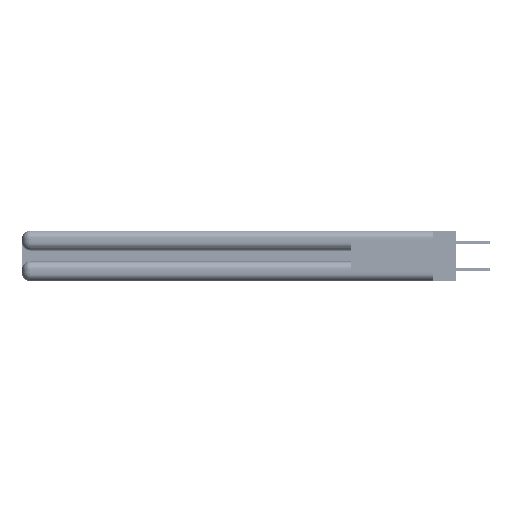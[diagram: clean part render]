
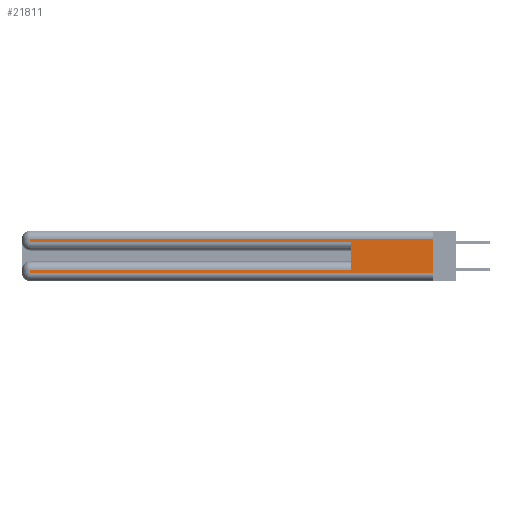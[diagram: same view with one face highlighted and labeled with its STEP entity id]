
A CAD part, left-side view. The second image highlights one B-rep face of the part: STEP entity #21811.
In plain terms, the highlighted planar face has unit normal (-1, 0, 0).
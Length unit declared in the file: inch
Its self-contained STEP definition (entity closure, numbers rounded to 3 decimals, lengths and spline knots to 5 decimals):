
#306 = VERTEX_POINT ( 'NONE', #36244 ) ;
#839 = CARTESIAN_POINT ( 'NONE',  ( 0., 2.94, 0.37 ) ) ;
#999 = VECTOR ( 'NONE', #22378, 39.37008 ) ;
#1964 = EDGE_CURVE ( 'NONE', #41503, #306, #30579, .T. ) ;
#2880 = CARTESIAN_POINT ( 'NONE',  ( 0., 2.94, 0.285 ) ) ;
#4609 = VECTOR ( 'NONE', #44066, 39.37008 ) ;
#4792 = VECTOR ( 'NONE', #18632, 39.37008 ) ;
#5187 = VERTEX_POINT ( 'NONE', #34090 ) ;
#5436 = CARTESIAN_POINT ( 'NONE',  ( 0., 2.94, 0.06 ) ) ;
#5549 = DIRECTION ( 'NONE',  ( 1., 0., 0. ) ) ;
#5707 = PLANE ( 'NONE',  #13235 ) ;
#6032 = EDGE_CURVE ( 'NONE', #41503, #29476, #15359, .T. ) ;
#6185 = FACE_OUTER_BOUND ( 'NONE', #9806, .T. ) ;
#6890 = LINE ( 'NONE', #13464, #4609 ) ;
#7035 = LINE ( 'NONE', #839, #19887 ) ;
#7807 = LINE ( 'NONE', #8711, #35092 ) ;
#8030 = DIRECTION ( 'NONE',  ( 0., 0., -1. ) ) ;
#8711 = CARTESIAN_POINT ( 'NONE',  ( 0., 0., 0.085 ) ) ;
#9121 = DIRECTION ( 'NONE',  ( 0., 0., -1. ) ) ;
#9806 = EDGE_LOOP ( 'NONE', ( #16525, #15407, #21273, #27551, #45612, #13527, #24434, #16816 ) ) ;
#9994 = VECTOR ( 'NONE', #25529, 39.37008 ) ;
#11656 = CARTESIAN_POINT ( 'NONE',  ( 0., 0., 0.37 ) ) ;
#12857 = CARTESIAN_POINT ( 'NONE',  ( 0., 0., 0.37 ) ) ;
#13235 = AXIS2_PLACEMENT_3D ( 'NONE', #12857, #5549, #9121 ) ;
#13464 = CARTESIAN_POINT ( 'NONE',  ( 0., 0.6, 0.145 ) ) ;
#13527 = ORIENTED_EDGE ( 'NONE', *, *, #14182, .T. ) ;
#14182 = EDGE_CURVE ( 'NONE', #41572, #17109, #7807, .T. ) ;
#14667 = CARTESIAN_POINT ( 'NONE',  ( 0., 0., 0.06 ) ) ;
#14694 = VERTEX_POINT ( 'NONE', #5436 ) ;
#15359 = LINE ( 'NONE', #22046, #4792 ) ;
#15407 = ORIENTED_EDGE ( 'NONE', *, *, #6032, .T. ) ;
#16525 = ORIENTED_EDGE ( 'NONE', *, *, #1964, .F. ) ;
#16552 = LINE ( 'NONE', #27959, #25923 ) ;
#16816 = ORIENTED_EDGE ( 'NONE', *, *, #29299, .T. ) ;
#16933 = DIRECTION ( 'NONE',  ( 0., 0., -1. ) ) ;
#17109 = VERTEX_POINT ( 'NONE', #32635 ) ;
#18632 = DIRECTION ( 'NONE',  ( 0., 1., 0. ) ) ;
#19887 = VECTOR ( 'NONE', #8030, 39.37008 ) ;
#20231 = EDGE_CURVE ( 'NONE', #41572, #5187, #6890, .T. ) ;
#21273 = ORIENTED_EDGE ( 'NONE', *, *, #32077, .T. ) ;
#21811 = ADVANCED_FACE ( 'NONE', ( #6185 ), #5707, .F. ) ;
#22046 = CARTESIAN_POINT ( 'NONE',  ( 0., 0., 0.31 ) ) ;
#22378 = DIRECTION ( 'NONE',  ( 0., 0., -1. ) ) ;
#24434 = ORIENTED_EDGE ( 'NONE', *, *, #35512, .T. ) ;
#24510 = DIRECTION ( 'NONE',  ( 0., -1., 0. ) ) ;
#25529 = DIRECTION ( 'NONE',  ( 0., -1., 0. ) ) ;
#25923 = VECTOR ( 'NONE', #24510, 39.37008 ) ;
#25929 = VERTEX_POINT ( 'NONE', #2880 ) ;
#26844 = CARTESIAN_POINT ( 'NONE',  ( 0., 2.94, 0.37 ) ) ;
#27551 = ORIENTED_EDGE ( 'NONE', *, *, #31058, .T. ) ;
#27959 = CARTESIAN_POINT ( 'NONE',  ( 0., 0., 0.285 ) ) ;
#28895 = LINE ( 'NONE', #14667, #9994 ) ;
#29275 = CARTESIAN_POINT ( 'NONE',  ( 0., 0.6, 0.085 ) ) ;
#29299 = EDGE_CURVE ( 'NONE', #14694, #306, #28895, .T. ) ;
#29476 = VERTEX_POINT ( 'NONE', #36619 ) ;
#30579 = LINE ( 'NONE', #11656, #999 ) ;
#30771 = LINE ( 'NONE', #26844, #32897 ) ;
#31058 = EDGE_CURVE ( 'NONE', #25929, #5187, #16552, .T. ) ;
#32077 = EDGE_CURVE ( 'NONE', #29476, #25929, #7035, .T. ) ;
#32084 = CARTESIAN_POINT ( 'NONE',  ( 0., 0., 0.31 ) ) ;
#32635 = CARTESIAN_POINT ( 'NONE',  ( 0., 2.94, 0.085 ) ) ;
#32897 = VECTOR ( 'NONE', #16933, 39.37008 ) ;
#34090 = CARTESIAN_POINT ( 'NONE',  ( 0., 0.6, 0.285 ) ) ;
#35092 = VECTOR ( 'NONE', #40304, 39.37008 ) ;
#35512 = EDGE_CURVE ( 'NONE', #17109, #14694, #30771, .T. ) ;
#36244 = CARTESIAN_POINT ( 'NONE',  ( 0., 0., 0.06 ) ) ;
#36619 = CARTESIAN_POINT ( 'NONE',  ( 0., 2.94, 0.31 ) ) ;
#40304 = DIRECTION ( 'NONE',  ( 0., 1., 0. ) ) ;
#41503 = VERTEX_POINT ( 'NONE', #32084 ) ;
#41572 = VERTEX_POINT ( 'NONE', #29275 ) ;
#44066 = DIRECTION ( 'NONE',  ( 0., 0., 1. ) ) ;
#45612 = ORIENTED_EDGE ( 'NONE', *, *, #20231, .F. ) ;
